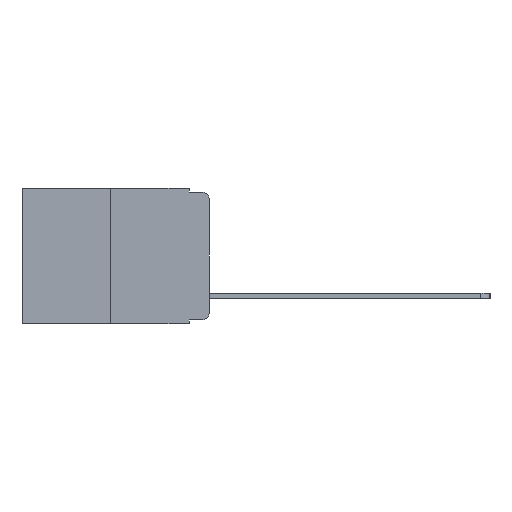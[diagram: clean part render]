
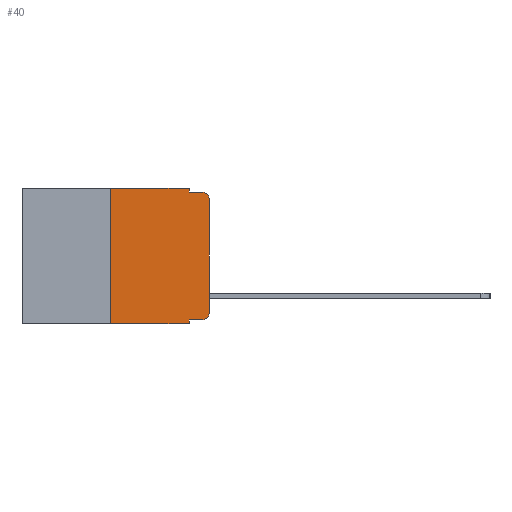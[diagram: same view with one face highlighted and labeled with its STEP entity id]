
A CAD part, left-side view. The second image highlights one B-rep face of the part: STEP entity #40.
In plain terms, the highlighted planar face has unit normal (-1, 0, 0).
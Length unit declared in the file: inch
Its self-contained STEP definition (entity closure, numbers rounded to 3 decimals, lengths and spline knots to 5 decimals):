
#40 = ADVANCED_FACE ( 'NONE', ( #5923 ), #4665, .F. ) ;
#201 = CARTESIAN_POINT ( 'NONE',  ( 0., 0.051, -0.01 ) ) ;
#262 = CARTESIAN_POINT ( 'NONE',  ( 0., 0.051, 0. ) ) ;
#290 = CIRCLE ( 'NONE', #12508, 0.02 ) ;
#332 = VECTOR ( 'NONE', #14011, 39.37008 ) ;
#423 = DIRECTION ( 'NONE',  ( 0., -1., 0. ) ) ;
#517 = EDGE_CURVE ( 'NONE', #10717, #12455, #1958, .T. ) ;
#614 = CARTESIAN_POINT ( 'NONE',  ( 0., 0.02, -0.313 ) ) ;
#649 = DIRECTION ( 'NONE',  ( 0., -1., 0. ) ) ;
#824 = ORIENTED_EDGE ( 'NONE', *, *, #1408, .F. ) ;
#1144 = CARTESIAN_POINT ( 'NONE',  ( 0., 0., 0. ) ) ;
#1176 = EDGE_CURVE ( 'NONE', #5029, #10902, #3606, .T. ) ;
#1357 = VECTOR ( 'NONE', #14331, 39.37008 ) ;
#1408 = EDGE_CURVE ( 'NONE', #6985, #10717, #12867, .T. ) ;
#1435 = ORIENTED_EDGE ( 'NONE', *, *, #517, .F. ) ;
#1460 = VERTEX_POINT ( 'NONE', #5516 ) ;
#1724 = EDGE_CURVE ( 'NONE', #6659, #6985, #3923, .T. ) ;
#1810 = CARTESIAN_POINT ( 'NONE',  ( 0., 0.02, -0.01 ) ) ;
#1904 = DIRECTION ( 'NONE',  ( 0., 0., -1. ) ) ;
#1958 = LINE ( 'NONE', #201, #4322 ) ;
#2007 = ORIENTED_EDGE ( 'NONE', *, *, #1176, .T. ) ;
#2102 = CARTESIAN_POINT ( 'NONE',  ( 0., 0.051, -0.333 ) ) ;
#2190 = EDGE_CURVE ( 'NONE', #5029, #6659, #4270, .T. ) ;
#2307 = CARTESIAN_POINT ( 'NONE',  ( 0., 0.25, 0. ) ) ;
#2309 = CARTESIAN_POINT ( 'NONE',  ( 0., 0.051, -0.343 ) ) ;
#2313 = DIRECTION ( 'NONE',  ( 0., 0., 1. ) ) ;
#2373 = DIRECTION ( 'NONE',  ( 0., 0., 1. ) ) ;
#2454 = CARTESIAN_POINT ( 'NONE',  ( 0., 0.473, 0. ) ) ;
#2687 = CARTESIAN_POINT ( 'NONE',  ( 0., 0.473, -0.343 ) ) ;
#2803 = DIRECTION ( 'NONE',  ( 0., 0., -1. ) ) ;
#3032 = EDGE_CURVE ( 'NONE', #3592, #10902, #12507, .T. ) ;
#3539 = CARTESIAN_POINT ( 'NONE',  ( 0., 0.051, 0. ) ) ;
#3592 = VERTEX_POINT ( 'NONE', #2102 ) ;
#3606 = LINE ( 'NONE', #2687, #332 ) ;
#3778 = EDGE_CURVE ( 'NONE', #3592, #1460, #9069, .T. ) ;
#3923 = LINE ( 'NONE', #2454, #12701 ) ;
#3969 = DIRECTION ( 'NONE',  ( 1., 0., 0. ) ) ;
#4074 = DIRECTION ( 'NONE',  ( 0., 0., -1. ) ) ;
#4089 = ORIENTED_EDGE ( 'NONE', *, *, #3032, .F. ) ;
#4237 = ORIENTED_EDGE ( 'NONE', *, *, #3778, .T. ) ;
#4270 = LINE ( 'NONE', #2307, #7315 ) ;
#4322 = VECTOR ( 'NONE', #9166, 39.37008 ) ;
#4527 = EDGE_CURVE ( 'NONE', #1460, #7593, #290, .T. ) ;
#4665 = PLANE ( 'NONE',  #9387 ) ;
#5029 = VERTEX_POINT ( 'NONE', #8686 ) ;
#5172 = ORIENTED_EDGE ( 'NONE', *, *, #4527, .T. ) ;
#5516 = CARTESIAN_POINT ( 'NONE',  ( 0., 0.02, -0.333 ) ) ;
#5923 = FACE_OUTER_BOUND ( 'NONE', #7495, .T. ) ;
#6317 = DIRECTION ( 'NONE',  ( -1., 0., 0. ) ) ;
#6659 = VERTEX_POINT ( 'NONE', #11800 ) ;
#6985 = VERTEX_POINT ( 'NONE', #3539 ) ;
#7315 = VECTOR ( 'NONE', #2313, 39.37008 ) ;
#7495 = EDGE_LOOP ( 'NONE', ( #10207, #8018, #1435, #824, #8930, #7517, #2007, #4089, #4237, #5172 ) ) ;
#7517 = ORIENTED_EDGE ( 'NONE', *, *, #2190, .F. ) ;
#7593 = VERTEX_POINT ( 'NONE', #9788 ) ;
#7873 = CARTESIAN_POINT ( 'NONE',  ( 0., 0.051, 0. ) ) ;
#8018 = ORIENTED_EDGE ( 'NONE', *, *, #14259, .T. ) ;
#8062 = CARTESIAN_POINT ( 'NONE',  ( 0., 0.051, -0.333 ) ) ;
#8686 = CARTESIAN_POINT ( 'NONE',  ( 0., 0.25, -0.343 ) ) ;
#8699 = CARTESIAN_POINT ( 'NONE',  ( 0., 0.051, -0.01 ) ) ;
#8749 = DIRECTION ( 'NONE',  ( -1., 0., 0. ) ) ;
#8918 = LINE ( 'NONE', #1144, #11461 ) ;
#8930 = ORIENTED_EDGE ( 'NONE', *, *, #1724, .F. ) ;
#9069 = LINE ( 'NONE', #8062, #11918 ) ;
#9166 = DIRECTION ( 'NONE',  ( 0., -1., 0. ) ) ;
#9387 = AXIS2_PLACEMENT_3D ( 'NONE', #13215, #3969, #4074 ) ;
#9731 = VECTOR ( 'NONE', #2803, 39.37008 ) ;
#9788 = CARTESIAN_POINT ( 'NONE',  ( 0., 0., -0.313 ) ) ;
#9839 = EDGE_CURVE ( 'NONE', #7593, #10266, #8918, .T. ) ;
#10207 = ORIENTED_EDGE ( 'NONE', *, *, #9839, .T. ) ;
#10266 = VERTEX_POINT ( 'NONE', #13338 ) ;
#10717 = VERTEX_POINT ( 'NONE', #8699 ) ;
#10902 = VERTEX_POINT ( 'NONE', #2309 ) ;
#11461 = VECTOR ( 'NONE', #2373, 39.37008 ) ;
#11589 = AXIS2_PLACEMENT_3D ( 'NONE', #12827, #6317, #13861 ) ;
#11800 = CARTESIAN_POINT ( 'NONE',  ( 0., 0.25, 0. ) ) ;
#11918 = VECTOR ( 'NONE', #649, 39.37008 ) ;
#12455 = VERTEX_POINT ( 'NONE', #1810 ) ;
#12507 = LINE ( 'NONE', #7873, #9731 ) ;
#12508 = AXIS2_PLACEMENT_3D ( 'NONE', #614, #8749, #1904 ) ;
#12701 = VECTOR ( 'NONE', #423, 39.37008 ) ;
#12827 = CARTESIAN_POINT ( 'NONE',  ( 0., 0.02, -0.03 ) ) ;
#12867 = LINE ( 'NONE', #262, #1357 ) ;
#13155 = CIRCLE ( 'NONE', #11589, 0.02 ) ;
#13215 = CARTESIAN_POINT ( 'NONE',  ( 0., 0.473, 0. ) ) ;
#13338 = CARTESIAN_POINT ( 'NONE',  ( 0., 0., -0.03 ) ) ;
#13861 = DIRECTION ( 'NONE',  ( 0., 0., -1. ) ) ;
#14011 = DIRECTION ( 'NONE',  ( 0., -1., 0. ) ) ;
#14259 = EDGE_CURVE ( 'NONE', #10266, #12455, #13155, .T. ) ;
#14331 = DIRECTION ( 'NONE',  ( 0., 0., -1. ) ) ;
